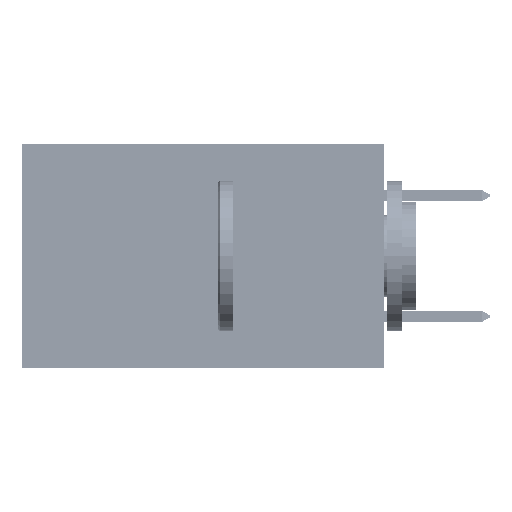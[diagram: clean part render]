
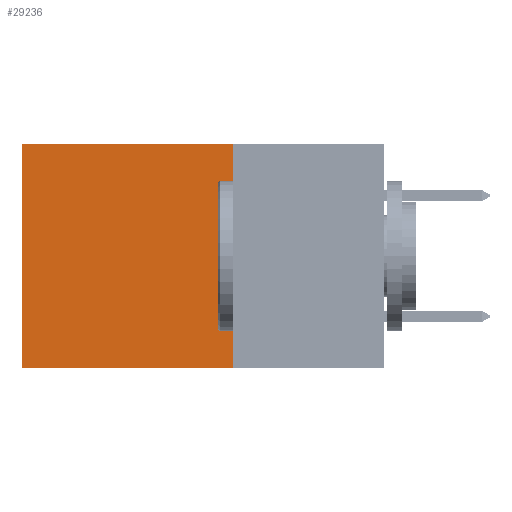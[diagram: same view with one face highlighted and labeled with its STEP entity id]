
A CAD part, left-side view. The second image highlights one B-rep face of the part: STEP entity #29236.
In plain terms, the highlighted planar face has unit normal (-1, 0, 0).
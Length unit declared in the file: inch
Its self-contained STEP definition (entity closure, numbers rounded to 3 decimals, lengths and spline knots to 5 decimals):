
#1374 = EDGE_CURVE ( 'NONE', #16638, #21598, #5340, .T. ) ;
#3212 = ORIENTED_EDGE ( 'NONE', *, *, #40729, .F. ) ;
#5340 = LINE ( 'NONE', #31455, #5931 ) ;
#5673 = ORIENTED_EDGE ( 'NONE', *, *, #30264, .T. ) ;
#5931 = VECTOR ( 'NONE', #36055, 39.37008 ) ;
#7294 = LINE ( 'NONE', #30785, #34817 ) ;
#7434 = FACE_OUTER_BOUND ( 'NONE', #43011, .T. ) ;
#11218 = CARTESIAN_POINT ( 'NONE',  ( 0.2875, 0.25, 0. ) ) ;
#11221 = VERTEX_POINT ( 'NONE', #34659 ) ;
#11912 = DIRECTION ( 'NONE',  ( 0., 1., 0. ) ) ;
#14756 = CARTESIAN_POINT ( 'NONE',  ( 0.2875, 0.25, -0.37 ) ) ;
#16638 = VERTEX_POINT ( 'NONE', #11218 ) ;
#18892 = DIRECTION ( 'NONE',  ( 0., 0., -1. ) ) ;
#19213 = PLANE ( 'NONE',  #23997 ) ;
#21543 = CARTESIAN_POINT ( 'NONE',  ( 0.2875, 0.6, 0. ) ) ;
#21598 = VERTEX_POINT ( 'NONE', #14756 ) ;
#23046 = ORIENTED_EDGE ( 'NONE', *, *, #1374, .F. ) ;
#23997 = AXIS2_PLACEMENT_3D ( 'NONE', #33881, #41197, #18892 ) ;
#26467 = ORIENTED_EDGE ( 'NONE', *, *, #39052, .T. ) ;
#26726 = CARTESIAN_POINT ( 'NONE',  ( 0.2875, 0.6, 0. ) ) ;
#29236 = ADVANCED_FACE ( 'NONE', ( #7434 ), #19213, .F. ) ;
#30264 = EDGE_CURVE ( 'NONE', #41696, #11221, #45667, .T. ) ;
#30462 = DIRECTION ( 'NONE',  ( 0., 1., 0. ) ) ;
#30785 = CARTESIAN_POINT ( 'NONE',  ( 0.2875, 0.25, -0.37 ) ) ;
#31455 = CARTESIAN_POINT ( 'NONE',  ( 0.2875, 0.25, 0. ) ) ;
#32781 = LINE ( 'NONE', #37296, #38485 ) ;
#33881 = CARTESIAN_POINT ( 'NONE',  ( 0.2875, 0.25, 0. ) ) ;
#34659 = CARTESIAN_POINT ( 'NONE',  ( 0.2875, 0.6, -0.37 ) ) ;
#34817 = VECTOR ( 'NONE', #30462, 39.37008 ) ;
#36055 = DIRECTION ( 'NONE',  ( 0., 0., -1. ) ) ;
#37081 = VECTOR ( 'NONE', #40006, 39.37008 ) ;
#37296 = CARTESIAN_POINT ( 'NONE',  ( 0.2875, 0.25, 0. ) ) ;
#38485 = VECTOR ( 'NONE', #11912, 39.37008 ) ;
#39052 = EDGE_CURVE ( 'NONE', #16638, #41696, #32781, .T. ) ;
#40006 = DIRECTION ( 'NONE',  ( 0., 0., -1. ) ) ;
#40729 = EDGE_CURVE ( 'NONE', #21598, #11221, #7294, .T. ) ;
#41197 = DIRECTION ( 'NONE',  ( 1., 0., 0. ) ) ;
#41696 = VERTEX_POINT ( 'NONE', #26726 ) ;
#43011 = EDGE_LOOP ( 'NONE', ( #5673, #3212, #23046, #26467 ) ) ;
#45667 = LINE ( 'NONE', #21543, #37081 ) ;
